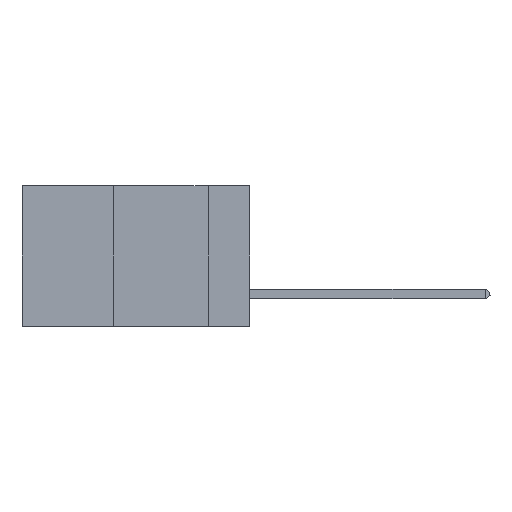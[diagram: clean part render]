
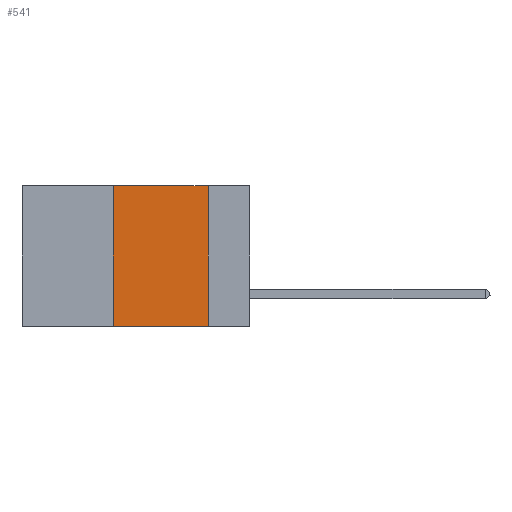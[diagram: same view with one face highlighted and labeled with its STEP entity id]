
A CAD part, left-side view. The second image highlights one B-rep face of the part: STEP entity #541.
In plain terms, the highlighted planar face has unit normal (-1, 0, 0).
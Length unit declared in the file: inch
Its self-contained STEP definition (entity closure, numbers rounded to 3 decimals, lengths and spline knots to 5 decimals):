
#345 = AXIS2_PLACEMENT_3D ( 'NONE', #4642, #15474, #12511 ) ;
#541 = ADVANCED_FACE ( 'NONE', ( #6854 ), #13932, .F. ) ;
#748 = VERTEX_POINT ( 'NONE', #19545 ) ;
#1050 = LINE ( 'NONE', #12634, #10210 ) ;
#2140 = VECTOR ( 'NONE', #15255, 39.37008 ) ;
#2326 = VERTEX_POINT ( 'NONE', #6721 ) ;
#2337 = DIRECTION ( 'NONE',  ( 0., -1., 0. ) ) ;
#3339 = CARTESIAN_POINT ( 'NONE',  ( 0., 0.11, 0. ) ) ;
#4642 = CARTESIAN_POINT ( 'NONE',  ( 0., 0.6, 0. ) ) ;
#4831 = DIRECTION ( 'NONE',  ( 0., 0., 1. ) ) ;
#5941 = EDGE_LOOP ( 'NONE', ( #19162, #8796, #16103, #17996 ) ) ;
#6568 = VERTEX_POINT ( 'NONE', #13552 ) ;
#6721 = CARTESIAN_POINT ( 'NONE',  ( 0., 0.11, -0.37 ) ) ;
#6854 = FACE_OUTER_BOUND ( 'NONE', #5941, .T. ) ;
#8091 = DIRECTION ( 'NONE',  ( 0., 0., -1. ) ) ;
#8796 = ORIENTED_EDGE ( 'NONE', *, *, #19180, .F. ) ;
#9885 = EDGE_CURVE ( 'NONE', #6568, #2326, #14456, .T. ) ;
#10210 = VECTOR ( 'NONE', #4831, 39.37008 ) ;
#12497 = EDGE_CURVE ( 'NONE', #6568, #13208, #1050, .T. ) ;
#12511 = DIRECTION ( 'NONE',  ( 0., 0., -1. ) ) ;
#12634 = CARTESIAN_POINT ( 'NONE',  ( 0., 0.36, 0. ) ) ;
#13208 = VERTEX_POINT ( 'NONE', #17959 ) ;
#13552 = CARTESIAN_POINT ( 'NONE',  ( 0., 0.36, -0.37 ) ) ;
#13825 = CARTESIAN_POINT ( 'NONE',  ( 0., 0.6, -0.37 ) ) ;
#13932 = PLANE ( 'NONE',  #345 ) ;
#14210 = LINE ( 'NONE', #3339, #16148 ) ;
#14456 = LINE ( 'NONE', #13825, #18087 ) ;
#14964 = EDGE_CURVE ( 'NONE', #748, #2326, #14210, .T. ) ;
#15255 = DIRECTION ( 'NONE',  ( 0., -1., 0. ) ) ;
#15474 = DIRECTION ( 'NONE',  ( 1., 0., 0. ) ) ;
#16103 = ORIENTED_EDGE ( 'NONE', *, *, #12497, .F. ) ;
#16148 = VECTOR ( 'NONE', #8091, 39.37008 ) ;
#17959 = CARTESIAN_POINT ( 'NONE',  ( 0., 0.36, 0. ) ) ;
#17996 = ORIENTED_EDGE ( 'NONE', *, *, #9885, .T. ) ;
#18087 = VECTOR ( 'NONE', #2337, 39.37008 ) ;
#19162 = ORIENTED_EDGE ( 'NONE', *, *, #14964, .F. ) ;
#19180 = EDGE_CURVE ( 'NONE', #13208, #748, #19747, .T. ) ;
#19377 = CARTESIAN_POINT ( 'NONE',  ( 0., 0.6, 0. ) ) ;
#19545 = CARTESIAN_POINT ( 'NONE',  ( 0., 0.11, 0. ) ) ;
#19747 = LINE ( 'NONE', #19377, #2140 ) ;
